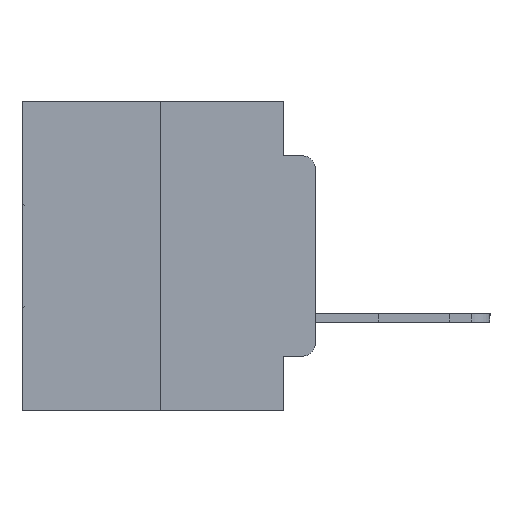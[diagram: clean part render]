
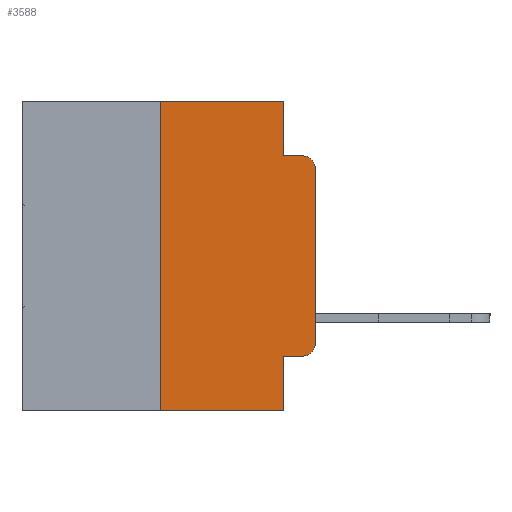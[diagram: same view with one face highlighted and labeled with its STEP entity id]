
A CAD part, left-side view. The second image highlights one B-rep face of the part: STEP entity #3588.
In plain terms, the highlighted planar face has unit normal (-1, 0, 0).
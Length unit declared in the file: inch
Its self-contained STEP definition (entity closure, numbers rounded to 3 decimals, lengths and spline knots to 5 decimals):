
#706 = LINE ( 'NONE', #26083, #12259 ) ;
#1271 = VERTEX_POINT ( 'NONE', #5362 ) ;
#1752 = VERTEX_POINT ( 'NONE', #4721 ) ;
#1885 = LINE ( 'NONE', #17984, #24663 ) ;
#1951 = VECTOR ( 'NONE', #16737, 39.37008 ) ;
#2188 = CARTESIAN_POINT ( 'NONE',  ( 0., 0.25, 0. ) ) ;
#3223 = EDGE_CURVE ( 'NONE', #18094, #18537, #17234, .T. ) ;
#3588 = ADVANCED_FACE ( 'NONE', ( #6581 ), #22556, .F. ) ;
#4183 = LINE ( 'NONE', #8695, #13483 ) ;
#4430 = DIRECTION ( 'NONE',  ( -1., 0., 0. ) ) ;
#4721 = CARTESIAN_POINT ( 'NONE',  ( 0., 0., -0.3915 ) ) ;
#5066 = VERTEX_POINT ( 'NONE', #25057 ) ;
#5163 = VECTOR ( 'NONE', #14499, 39.37008 ) ;
#5362 = CARTESIAN_POINT ( 'NONE',  ( 0., 0.051, 0. ) ) ;
#5597 = CIRCLE ( 'NONE', #13384, 0.02 ) ;
#6112 = LINE ( 'NONE', #9012, #16055 ) ;
#6581 = FACE_OUTER_BOUND ( 'NONE', #20757, .T. ) ;
#7163 = CARTESIAN_POINT ( 'NONE',  ( 0., 0.25, -0.5 ) ) ;
#7179 = ORIENTED_EDGE ( 'NONE', *, *, #17127, .F. ) ;
#7932 = VERTEX_POINT ( 'NONE', #17363 ) ;
#8054 = EDGE_CURVE ( 'NONE', #5066, #1752, #16799, .T. ) ;
#8695 = CARTESIAN_POINT ( 'NONE',  ( 0., 0.051, -0.4115 ) ) ;
#9009 = DIRECTION ( 'NONE',  ( -1., 0., 0. ) ) ;
#9012 = CARTESIAN_POINT ( 'NONE',  ( 0., 0., 0. ) ) ;
#9088 = EDGE_CURVE ( 'NONE', #11233, #1271, #25936, .T. ) ;
#9420 = CARTESIAN_POINT ( 'NONE',  ( 0., 0., -0.1085 ) ) ;
#9727 = ORIENTED_EDGE ( 'NONE', *, *, #11093, .T. ) ;
#11093 = EDGE_CURVE ( 'NONE', #24736, #5066, #4183, .T. ) ;
#11096 = ORIENTED_EDGE ( 'NONE', *, *, #26231, .T. ) ;
#11097 = VECTOR ( 'NONE', #12737, 39.37008 ) ;
#11233 = VERTEX_POINT ( 'NONE', #2188 ) ;
#11272 = DIRECTION ( 'NONE',  ( 0., 0., -1. ) ) ;
#11313 = DIRECTION ( 'NONE',  ( 0., 0., -1. ) ) ;
#11314 = CARTESIAN_POINT ( 'NONE',  ( 0., 0.051, -0.0885 ) ) ;
#12231 = CARTESIAN_POINT ( 'NONE',  ( 0., 0.473, -0.5 ) ) ;
#12259 = VECTOR ( 'NONE', #28358, 39.37008 ) ;
#12674 = DIRECTION ( 'NONE',  ( 0., -1., 0. ) ) ;
#12737 = DIRECTION ( 'NONE',  ( 0., 0., 1. ) ) ;
#13384 = AXIS2_PLACEMENT_3D ( 'NONE', #18048, #4430, #20309 ) ;
#13483 = VECTOR ( 'NONE', #24464, 39.37008 ) ;
#14122 = EDGE_CURVE ( 'NONE', #24736, #18537, #706, .T. ) ;
#14146 = LINE ( 'NONE', #25728, #1951 ) ;
#14499 = DIRECTION ( 'NONE',  ( 0., -1., 0. ) ) ;
#15005 = ORIENTED_EDGE ( 'NONE', *, *, #14122, .F. ) ;
#15360 = AXIS2_PLACEMENT_3D ( 'NONE', #29302, #24834, #11313 ) ;
#15628 = EDGE_CURVE ( 'NONE', #18094, #11233, #17805, .T. ) ;
#16055 = VECTOR ( 'NONE', #27174, 39.37008 ) ;
#16509 = CARTESIAN_POINT ( 'NONE',  ( 0., 0.051, -0.4115 ) ) ;
#16737 = DIRECTION ( 'NONE',  ( 0., -1., 0. ) ) ;
#16799 = CIRCLE ( 'NONE', #22617, 0.02 ) ;
#17127 = EDGE_CURVE ( 'NONE', #1271, #20325, #1885, .T. ) ;
#17198 = CARTESIAN_POINT ( 'NONE',  ( 0., 0.473, 0. ) ) ;
#17221 = VERTEX_POINT ( 'NONE', #9420 ) ;
#17234 = LINE ( 'NONE', #12231, #5163 ) ;
#17363 = CARTESIAN_POINT ( 'NONE',  ( 0., 0.02, -0.0885 ) ) ;
#17805 = LINE ( 'NONE', #21698, #11097 ) ;
#17984 = CARTESIAN_POINT ( 'NONE',  ( 0., 0.051, 0. ) ) ;
#18048 = CARTESIAN_POINT ( 'NONE',  ( 0., 0.02, -0.1085 ) ) ;
#18094 = VERTEX_POINT ( 'NONE', #7163 ) ;
#18537 = VERTEX_POINT ( 'NONE', #22244 ) ;
#18877 = ORIENTED_EDGE ( 'NONE', *, *, #3223, .T. ) ;
#20309 = DIRECTION ( 'NONE',  ( 0., 0., -1. ) ) ;
#20325 = VERTEX_POINT ( 'NONE', #11314 ) ;
#20757 = EDGE_LOOP ( 'NONE', ( #11096, #23090, #23792, #7179, #21345, #27386, #18877, #15005, #9727, #23814 ) ) ;
#21345 = ORIENTED_EDGE ( 'NONE', *, *, #9088, .F. ) ;
#21666 = EDGE_CURVE ( 'NONE', #20325, #7932, #14146, .T. ) ;
#21698 = CARTESIAN_POINT ( 'NONE',  ( 0., 0.25, 0. ) ) ;
#22244 = CARTESIAN_POINT ( 'NONE',  ( 0., 0.051, -0.5 ) ) ;
#22496 = CARTESIAN_POINT ( 'NONE',  ( 0., 0.02, -0.3915 ) ) ;
#22556 = PLANE ( 'NONE',  #15360 ) ;
#22617 = AXIS2_PLACEMENT_3D ( 'NONE', #22496, #9009, #24764 ) ;
#23090 = ORIENTED_EDGE ( 'NONE', *, *, #23189, .T. ) ;
#23189 = EDGE_CURVE ( 'NONE', #17221, #7932, #5597, .T. ) ;
#23792 = ORIENTED_EDGE ( 'NONE', *, *, #21666, .F. ) ;
#23814 = ORIENTED_EDGE ( 'NONE', *, *, #8054, .T. ) ;
#24464 = DIRECTION ( 'NONE',  ( 0., -1., 0. ) ) ;
#24663 = VECTOR ( 'NONE', #11272, 39.37008 ) ;
#24736 = VERTEX_POINT ( 'NONE', #16509 ) ;
#24764 = DIRECTION ( 'NONE',  ( 0., 0., -1. ) ) ;
#24834 = DIRECTION ( 'NONE',  ( 1., 0., 0. ) ) ;
#25057 = CARTESIAN_POINT ( 'NONE',  ( 0., 0.02, -0.4115 ) ) ;
#25212 = VECTOR ( 'NONE', #12674, 39.37008 ) ;
#25728 = CARTESIAN_POINT ( 'NONE',  ( 0., 0.051, -0.0885 ) ) ;
#25936 = LINE ( 'NONE', #17198, #25212 ) ;
#26083 = CARTESIAN_POINT ( 'NONE',  ( 0., 0.051, 0. ) ) ;
#26231 = EDGE_CURVE ( 'NONE', #1752, #17221, #6112, .T. ) ;
#27174 = DIRECTION ( 'NONE',  ( 0., 0., 1. ) ) ;
#27386 = ORIENTED_EDGE ( 'NONE', *, *, #15628, .F. ) ;
#28358 = DIRECTION ( 'NONE',  ( 0., 0., -1. ) ) ;
#29302 = CARTESIAN_POINT ( 'NONE',  ( 0., 0.473, 0. ) ) ;
